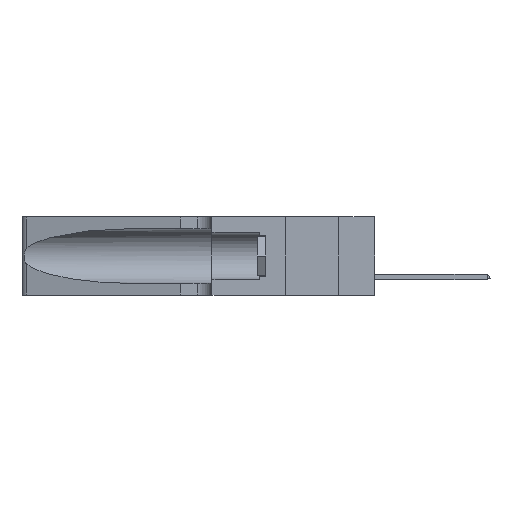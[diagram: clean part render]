
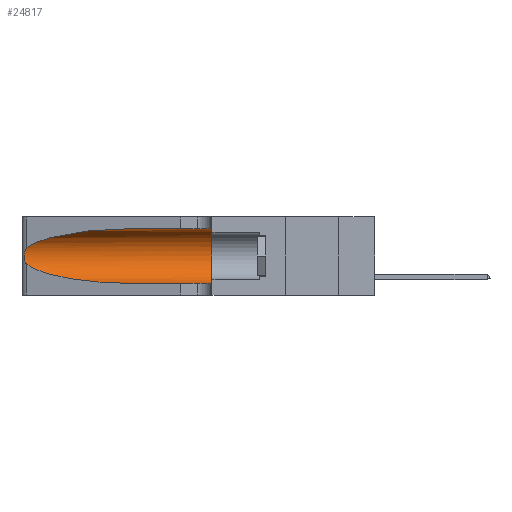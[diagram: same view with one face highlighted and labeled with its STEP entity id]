
A CAD part, left-side view. The second image highlights one B-rep face of the part: STEP entity #24817.
In plain terms, the highlighted cylindrical face has radius 3.308 mm (diameter 6.617 mm), a partial arc.
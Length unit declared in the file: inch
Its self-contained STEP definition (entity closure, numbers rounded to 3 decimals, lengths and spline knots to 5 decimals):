
#792 = CARTESIAN_POINT ( 'NONE',  ( 0.1305, 0.72297, 0.31525 ) ) ;
#895 = DIRECTION ( 'NONE',  ( 0., 0., -1. ) ) ;
#1082 = CARTESIAN_POINT ( 'NONE',  ( 0.25854, 1.2359, 0.20912 ) ) ;
#1655 = VERTEX_POINT ( 'NONE', #6482 ) ;
#2581 = CARTESIAN_POINT ( 'NONE',  ( 0.25487, 1.22718, 0.14631 ) ) ;
#2887 = AXIS2_PLACEMENT_3D ( 'NONE', #14322, #14508, #895 ) ;
#3085 = DIRECTION ( 'NONE',  ( 0., -1., 0. ) ) ;
#3262 = DIRECTION ( 'NONE',  ( 0., 1., 0. ) ) ;
#3336 = ORIENTED_EDGE ( 'NONE', *, *, #22710, .T. ) ;
#3479 = CARTESIAN_POINT ( 'NONE',  ( 0.26075, 1.23896, 0.19203 ) ) ;
#4369 = ORIENTED_EDGE ( 'NONE', *, *, #7751, .T. ) ;
#4534 = CARTESIAN_POINT ( 'NONE',  ( 0.1305, 0.72297, 0.31525 ) ) ;
#6008 = CARTESIAN_POINT ( 'NONE',  ( 0.25787, 1.23484, 0.2124 ) ) ;
#6116 = CARTESIAN_POINT ( 'NONE',  ( 0.25789, 1.23486, 0.15765 ) ) ;
#6482 = CARTESIAN_POINT ( 'NONE',  ( 0.1305, 0.35, 0.31525 ) ) ;
#6742 = VERTEX_POINT ( 'NONE', #20927 ) ;
#7144 = CYLINDRICAL_SURFACE ( 'NONE', #2887, 0.13025 ) ;
#7541 = VERTEX_POINT ( 'NONE', #13121 ) ;
#7751 = EDGE_CURVE ( 'NONE', #24843, #7541, #22650, .T. ) ;
#8112 = CARTESIAN_POINT ( 'NONE',  ( 0.25856, 1.23593, 0.16098 ) ) ;
#8222 = ORIENTED_EDGE ( 'NONE', *, *, #9105, .F. ) ;
#8297 = CARTESIAN_POINT ( 'NONE',  ( 0.25487, 1.22718, 0.14631 ) ) ;
#8588 = ORIENTED_EDGE ( 'NONE', *, *, #25398, .F. ) ;
#8615 = ORIENTED_EDGE ( 'NONE', *, *, #9449, .T. ) ;
#9105 = EDGE_CURVE ( 'NONE', #24843, #1655, #19107, .T. ) ;
#9325 = CARTESIAN_POINT ( 'NONE',  ( 0.1305, 0.72297, 0.05475 ) ) ;
#9449 = EDGE_CURVE ( 'NONE', #7541, #25480, #17342, .T. ) ;
#9546 = CARTESIAN_POINT ( 'NONE',  ( 0.1305, 1.61858, 0.05475 ) ) ;
#10299 = ORIENTED_EDGE ( 'NONE', *, *, #21350, .T. ) ;
#11249 = CARTESIAN_POINT ( 'NONE',  ( 0.18966, 0.96281, 0.31525 ) ) ;
#11640 = LINE ( 'NONE', #9546, #19814 ) ;
#12709 = CARTESIAN_POINT ( 'NONE',  ( 0.25555, 1.22993, 0.14849 ) ) ;
#13121 = CARTESIAN_POINT ( 'NONE',  ( 0.25487, 1.22718, 0.22369 ) ) ;
#14007 = CARTESIAN_POINT ( 'NONE',  ( 0.1305, 0.35, 0.185 ) ) ;
#14322 = CARTESIAN_POINT ( 'NONE',  ( 0.1305, 1.61858, 0.185 ) ) ;
#14508 = DIRECTION ( 'NONE',  ( 0., -1., 0. ) ) ;
#14623 = FACE_OUTER_BOUND ( 'NONE', #24856, .T. ) ;
#15203 = CARTESIAN_POINT ( 'NONE',  ( 0.25487, 1.22718, 0.14631 ) ) ;
#16492 = CARTESIAN_POINT ( 'NONE',  ( 0.1305, 0.72297, 0.05475 ) ) ;
#16716 = DIRECTION ( 'NONE',  ( 0., 0., 1. ) ) ;
#17097 = CARTESIAN_POINT ( 'NONE',  ( 0.26017, 1.23833, 0.17102 ) ) ;
#17139 = VERTEX_POINT ( 'NONE', #16492 ) ;
#17342 = B_SPLINE_CURVE_WITH_KNOTS ( 'NONE', 3,
 ( #28753, #21863, #28853, #6008, #1082, #21652, #3479, #19473, #17097, #8112, #6116, #26241, #12709, #15203 ),
 .UNSPECIFIED., .F., .F.,
 ( 4, 2, 2, 2, 2, 2, 4 ),
 ( 0., 0.00027, 0.00053, 0.00107, 0.0016, 0.00187, 0.00214 ),
 .UNSPECIFIED. ) ;
#17418 =( BOUNDED_CURVE ( )  B_SPLINE_CURVE ( 3, ( #2581, #25335, #22969, #9325 ),
 .UNSPECIFIED., .F., .F. ) 
 B_SPLINE_CURVE_WITH_KNOTS ( ( 4, 4 ),
 ( 3.44316, 4.71239 ),
 .UNSPECIFIED. ) 
 CURVE ( )  GEOMETRIC_REPRESENTATION_ITEM ( )  RATIONAL_B_SPLINE_CURVE ( ( 1., 0.87, 0.87, 1. ) ) 
 REPRESENTATION_ITEM ( '' )  );
#19107 = LINE ( 'NONE', #21351, #21252 ) ;
#19473 = CARTESIAN_POINT ( 'NONE',  ( 0.26075, 1.23896, 0.178 ) ) ;
#19814 = VECTOR ( 'NONE', #3085, 39.37008 ) ;
#20508 = CARTESIAN_POINT ( 'NONE',  ( 0.2373, 1.15595, 0.28018 ) ) ;
#20927 = CARTESIAN_POINT ( 'NONE',  ( 0.1305, 0.35, 0.05475 ) ) ;
#21252 = VECTOR ( 'NONE', #23659, 39.37008 ) ;
#21350 = EDGE_CURVE ( 'NONE', #17139, #6742, #11640, .T. ) ;
#21351 = CARTESIAN_POINT ( 'NONE',  ( 0.1305, 1.61858, 0.31525 ) ) ;
#21352 = CIRCLE ( 'NONE', #22817, 0.13025 ) ;
#21652 = CARTESIAN_POINT ( 'NONE',  ( 0.26018, 1.23835, 0.19895 ) ) ;
#21863 = CARTESIAN_POINT ( 'NONE',  ( 0.25555, 1.22994, 0.2215 ) ) ;
#22650 =( BOUNDED_CURVE ( )  B_SPLINE_CURVE ( 3, ( #4534, #11249, #20508, #22809 ),
 .UNSPECIFIED., .F., .F. ) 
 B_SPLINE_CURVE_WITH_KNOTS ( ( 4, 4 ),
 ( 1.5708, 2.84003 ),
 .UNSPECIFIED. ) 
 CURVE ( )  GEOMETRIC_REPRESENTATION_ITEM ( )  RATIONAL_B_SPLINE_CURVE ( ( 1., 0.87, 0.87, 1. ) ) 
 REPRESENTATION_ITEM ( '' )  );
#22710 = EDGE_CURVE ( 'NONE', #25480, #17139, #17418, .T. ) ;
#22809 = CARTESIAN_POINT ( 'NONE',  ( 0.25487, 1.22718, 0.22369 ) ) ;
#22817 = AXIS2_PLACEMENT_3D ( 'NONE', #14007, #3262, #16716 ) ;
#22969 = CARTESIAN_POINT ( 'NONE',  ( 0.18966, 0.96281, 0.05475 ) ) ;
#23659 = DIRECTION ( 'NONE',  ( 0., -1., 0. ) ) ;
#24817 = ADVANCED_FACE ( 'NONE', ( #14623 ), #7144, .F. ) ;
#24843 = VERTEX_POINT ( 'NONE', #792 ) ;
#24856 = EDGE_LOOP ( 'NONE', ( #4369, #8615, #3336, #10299, #8588, #8222 ) ) ;
#25335 = CARTESIAN_POINT ( 'NONE',  ( 0.2373, 1.15595, 0.08982 ) ) ;
#25398 = EDGE_CURVE ( 'NONE', #1655, #6742, #21352, .T. ) ;
#25480 = VERTEX_POINT ( 'NONE', #8297 ) ;
#26241 = CARTESIAN_POINT ( 'NONE',  ( 0.25639, 1.23186, 0.15144 ) ) ;
#28753 = CARTESIAN_POINT ( 'NONE',  ( 0.25487, 1.22718, 0.22369 ) ) ;
#28853 = CARTESIAN_POINT ( 'NONE',  ( 0.25639, 1.23184, 0.21858 ) ) ;
